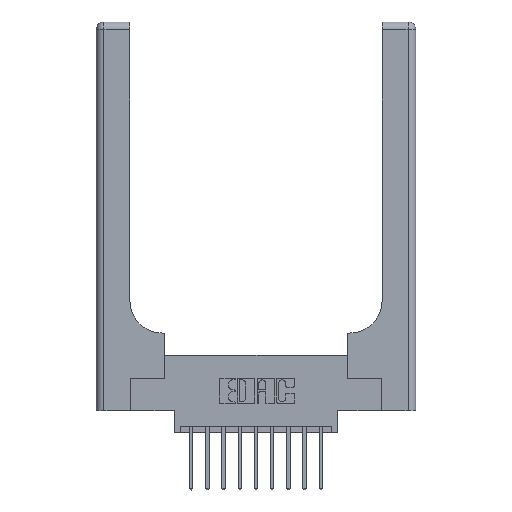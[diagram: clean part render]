
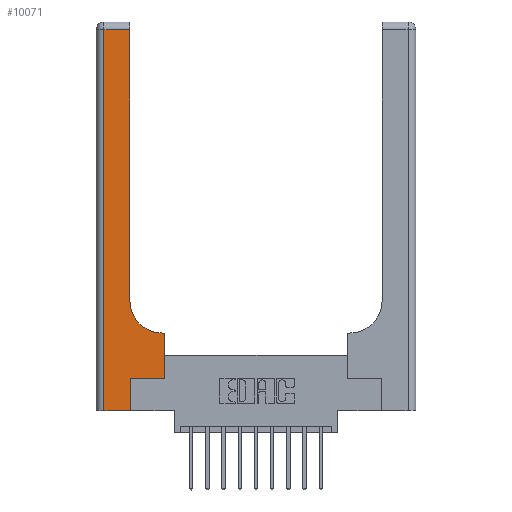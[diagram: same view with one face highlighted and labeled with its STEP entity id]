
A CAD part, top view. The second image highlights one B-rep face of the part: STEP entity #10071.
In plain terms, the highlighted planar face has unit normal (0, 0, 1).
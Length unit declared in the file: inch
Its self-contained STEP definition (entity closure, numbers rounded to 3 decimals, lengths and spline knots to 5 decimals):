
#431 = ORIENTED_EDGE ( 'NONE', *, *, #10337, .T. ) ;
#437 = VECTOR ( 'NONE', #9379, 39.37008 ) ;
#599 = VECTOR ( 'NONE', #14986, 39.37008 ) ;
#962 = CARTESIAN_POINT ( 'NONE',  ( 0.51, 0.85, 0.37 ) ) ;
#1158 = CARTESIAN_POINT ( 'NONE',  ( 0.265, 0.25, 0.37 ) ) ;
#1356 = LINE ( 'NONE', #3612, #13862 ) ;
#1454 = VERTEX_POINT ( 'NONE', #1158 ) ;
#1524 = DIRECTION ( 'NONE',  ( 0., 0., -1. ) ) ;
#1626 = CARTESIAN_POINT ( 'NONE',  ( 0.26, 0.6, 0.37 ) ) ;
#1686 = VECTOR ( 'NONE', #3714, 39.37008 ) ;
#1713 = CIRCLE ( 'NONE', #8645, 0.25 ) ;
#1742 = VERTEX_POINT ( 'NONE', #4156 ) ;
#2153 = ORIENTED_EDGE ( 'NONE', *, *, #7467, .T. ) ;
#2183 = DIRECTION ( 'NONE',  ( 1., 0., 0. ) ) ;
#2493 = LINE ( 'NONE', #5736, #14971 ) ;
#2773 = EDGE_LOOP ( 'NONE', ( #8343, #14281, #2153, #12236, #12594, #3285, #431, #4411, #4788 ) ) ;
#3023 = LINE ( 'NONE', #8501, #5906 ) ;
#3236 = CARTESIAN_POINT ( 'NONE',  ( 0.06, 3., 0.37 ) ) ;
#3285 = ORIENTED_EDGE ( 'NONE', *, *, #13276, .T. ) ;
#3316 = EDGE_CURVE ( 'NONE', #12103, #1742, #3663, .T. ) ;
#3390 = DIRECTION ( 'NONE',  ( 0., -1., 0. ) ) ;
#3418 = AXIS2_PLACEMENT_3D ( 'NONE', #14791, #1524, #10024 ) ;
#3612 = CARTESIAN_POINT ( 'NONE',  ( 0.265, 0., 0.37 ) ) ;
#3663 = LINE ( 'NONE', #11766, #437 ) ;
#3714 = DIRECTION ( 'NONE',  ( -1., 0., 0. ) ) ;
#3748 = VERTEX_POINT ( 'NONE', #4037 ) ;
#3940 = CARTESIAN_POINT ( 'NONE',  ( 0.06, 2.94, 0.37 ) ) ;
#4037 = CARTESIAN_POINT ( 'NONE',  ( 0.528, 0.6, 0.37 ) ) ;
#4156 = CARTESIAN_POINT ( 'NONE',  ( 0.26, 2.94, 0.37 ) ) ;
#4411 = ORIENTED_EDGE ( 'NONE', *, *, #11750, .T. ) ;
#4788 = ORIENTED_EDGE ( 'NONE', *, *, #13142, .T. ) ;
#4836 = EDGE_CURVE ( 'NONE', #6954, #13107, #2493, .T. ) ;
#5658 = LINE ( 'NONE', #3236, #12121 ) ;
#5736 = CARTESIAN_POINT ( 'NONE',  ( 0., 0., 0.37 ) ) ;
#5767 = LINE ( 'NONE', #5822, #7857 ) ;
#5822 = CARTESIAN_POINT ( 'NONE',  ( 0.528, 0.25, 0.37 ) ) ;
#5906 = VECTOR ( 'NONE', #10897, 39.37008 ) ;
#6366 = EDGE_CURVE ( 'NONE', #1742, #8744, #14931, .T. ) ;
#6954 = VERTEX_POINT ( 'NONE', #9666 ) ;
#6984 = DIRECTION ( 'NONE',  ( 1., 0., 0. ) ) ;
#7066 = DIRECTION ( 'NONE',  ( 0., 1., 0. ) ) ;
#7467 = EDGE_CURVE ( 'NONE', #8744, #6954, #5658, .T. ) ;
#7857 = VECTOR ( 'NONE', #7066, 39.37008 ) ;
#8343 = ORIENTED_EDGE ( 'NONE', *, *, #3316, .T. ) ;
#8501 = CARTESIAN_POINT ( 'NONE',  ( 0.265, 0.25, 0.37 ) ) ;
#8645 = AXIS2_PLACEMENT_3D ( 'NONE', #962, #9469, #2183 ) ;
#8744 = VERTEX_POINT ( 'NONE', #3940 ) ;
#8788 = PLANE ( 'NONE',  #3418 ) ;
#9379 = DIRECTION ( 'NONE',  ( 0., 1., 0. ) ) ;
#9469 = DIRECTION ( 'NONE',  ( 0., 0., -1. ) ) ;
#9666 = CARTESIAN_POINT ( 'NONE',  ( 0.06, 0., 0.37 ) ) ;
#9789 = CARTESIAN_POINT ( 'NONE',  ( 0.26, 0.85, 0.37 ) ) ;
#10024 = DIRECTION ( 'NONE',  ( -1., 0., 0. ) ) ;
#10071 = ADVANCED_FACE ( 'NONE', ( #10906 ), #8788, .F. ) ;
#10337 = EDGE_CURVE ( 'NONE', #14472, #3748, #5767, .T. ) ;
#10586 = CARTESIAN_POINT ( 'NONE',  ( 0.265, 0., 0.37 ) ) ;
#10897 = DIRECTION ( 'NONE',  ( 1., 0., 0. ) ) ;
#10906 = FACE_OUTER_BOUND ( 'NONE', #2773, .T. ) ;
#11025 = CARTESIAN_POINT ( 'NONE',  ( 0.528, 0.25, 0.37 ) ) ;
#11750 = EDGE_CURVE ( 'NONE', #3748, #13970, #14627, .T. ) ;
#11766 = CARTESIAN_POINT ( 'NONE',  ( 0.26, 3., 0.37 ) ) ;
#12103 = VERTEX_POINT ( 'NONE', #9789 ) ;
#12121 = VECTOR ( 'NONE', #3390, 39.37008 ) ;
#12236 = ORIENTED_EDGE ( 'NONE', *, *, #4836, .T. ) ;
#12594 = ORIENTED_EDGE ( 'NONE', *, *, #12654, .T. ) ;
#12654 = EDGE_CURVE ( 'NONE', #13107, #1454, #1356, .T. ) ;
#13107 = VERTEX_POINT ( 'NONE', #10586 ) ;
#13142 = EDGE_CURVE ( 'NONE', #13970, #12103, #1713, .T. ) ;
#13276 = EDGE_CURVE ( 'NONE', #1454, #14472, #3023, .T. ) ;
#13338 = DIRECTION ( 'NONE',  ( 0., 1., 0. ) ) ;
#13428 = CARTESIAN_POINT ( 'NONE',  ( 0., 2.94, 0.37 ) ) ;
#13862 = VECTOR ( 'NONE', #13338, 39.37008 ) ;
#13970 = VERTEX_POINT ( 'NONE', #14952 ) ;
#14281 = ORIENTED_EDGE ( 'NONE', *, *, #6366, .T. ) ;
#14472 = VERTEX_POINT ( 'NONE', #11025 ) ;
#14627 = LINE ( 'NONE', #1626, #599 ) ;
#14791 = CARTESIAN_POINT ( 'NONE',  ( 0., 3., 0.37 ) ) ;
#14931 = LINE ( 'NONE', #13428, #1686 ) ;
#14952 = CARTESIAN_POINT ( 'NONE',  ( 0.51, 0.6, 0.37 ) ) ;
#14971 = VECTOR ( 'NONE', #6984, 39.37008 ) ;
#14986 = DIRECTION ( 'NONE',  ( -1., 0., 0. ) ) ;
